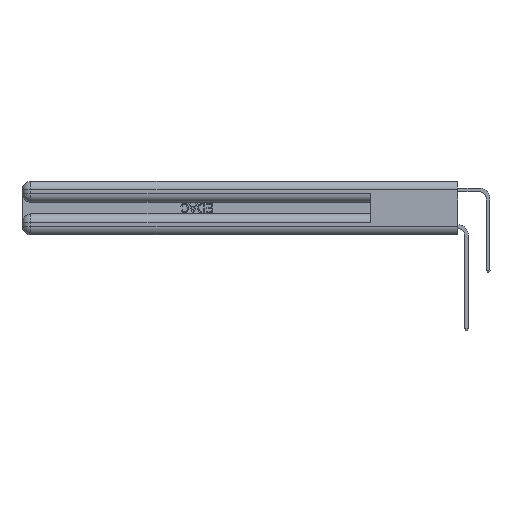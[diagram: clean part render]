
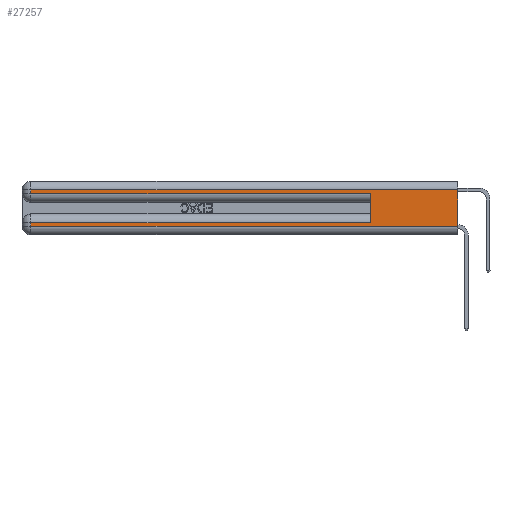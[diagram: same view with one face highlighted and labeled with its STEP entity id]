
A CAD part, left-side view. The second image highlights one B-rep face of the part: STEP entity #27257.
In plain terms, the highlighted planar face has unit normal (-1, 0, 0).
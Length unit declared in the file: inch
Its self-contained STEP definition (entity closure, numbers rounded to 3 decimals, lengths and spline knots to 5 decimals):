
#661 = VERTEX_POINT ( 'NONE', #8193 ) ;
#1344 = VERTEX_POINT ( 'NONE', #17011 ) ;
#1753 = CARTESIAN_POINT ( 'NONE',  ( 0., 2.94, 0.37 ) ) ;
#2162 = ORIENTED_EDGE ( 'NONE', *, *, #30334, .F. ) ;
#3228 = VECTOR ( 'NONE', #27298, 39.37008 ) ;
#3565 = VERTEX_POINT ( 'NONE', #12683 ) ;
#4190 = ORIENTED_EDGE ( 'NONE', *, *, #29912, .T. ) ;
#4237 = LINE ( 'NONE', #1753, #13322 ) ;
#4290 = CARTESIAN_POINT ( 'NONE',  ( 0., 0., 0.37 ) ) ;
#4573 = CARTESIAN_POINT ( 'NONE',  ( 0., 0.6, 0.285 ) ) ;
#5246 = CARTESIAN_POINT ( 'NONE',  ( 0., 2.94, 0.31 ) ) ;
#5286 = AXIS2_PLACEMENT_3D ( 'NONE', #32133, #14847, #19780 ) ;
#5303 = LINE ( 'NONE', #10839, #9142 ) ;
#5485 = CARTESIAN_POINT ( 'NONE',  ( 0., 0., 0.285 ) ) ;
#6929 = CARTESIAN_POINT ( 'NONE',  ( 0., 0., 0.31 ) ) ;
#7421 = CARTESIAN_POINT ( 'NONE',  ( 0., 0., 0.085 ) ) ;
#8007 = VERTEX_POINT ( 'NONE', #24613 ) ;
#8073 = ORIENTED_EDGE ( 'NONE', *, *, #30149, .T. ) ;
#8193 = CARTESIAN_POINT ( 'NONE',  ( 0., 0., 0.06 ) ) ;
#9142 = VECTOR ( 'NONE', #25018, 39.37008 ) ;
#10044 = DIRECTION ( 'NONE',  ( 0., 1., 0. ) ) ;
#10587 = VERTEX_POINT ( 'NONE', #27217 ) ;
#10736 = FACE_OUTER_BOUND ( 'NONE', #17680, .T. ) ;
#10839 = CARTESIAN_POINT ( 'NONE',  ( 0., 0.6, 0.145 ) ) ;
#11216 = EDGE_CURVE ( 'NONE', #8007, #10587, #24438, .T. ) ;
#11605 = VECTOR ( 'NONE', #14109, 39.37008 ) ;
#11697 = CARTESIAN_POINT ( 'NONE',  ( 0., 0., 0.06 ) ) ;
#12253 = PLANE ( 'NONE',  #5286 ) ;
#12683 = CARTESIAN_POINT ( 'NONE',  ( 0., 0., 0.31 ) ) ;
#12942 = VECTOR ( 'NONE', #24600, 39.37008 ) ;
#13322 = VECTOR ( 'NONE', #16979, 39.37008 ) ;
#14109 = DIRECTION ( 'NONE',  ( 0., -1., 0. ) ) ;
#14599 = LINE ( 'NONE', #11697, #11605 ) ;
#14847 = DIRECTION ( 'NONE',  ( 1., 0., 0. ) ) ;
#16370 = EDGE_CURVE ( 'NONE', #28521, #16563, #4237, .T. ) ;
#16563 = VERTEX_POINT ( 'NONE', #27838 ) ;
#16886 = LINE ( 'NONE', #4290, #25620 ) ;
#16979 = DIRECTION ( 'NONE',  ( 0., 0., -1. ) ) ;
#17011 = CARTESIAN_POINT ( 'NONE',  ( 0., 0.6, 0.085 ) ) ;
#17680 = EDGE_LOOP ( 'NONE', ( #17931, #8073, #31713, #4190, #2162, #29320, #31183, #22426 ) ) ;
#17931 = ORIENTED_EDGE ( 'NONE', *, *, #22039, .F. ) ;
#18615 = VECTOR ( 'NONE', #10044, 39.37008 ) ;
#19661 = VECTOR ( 'NONE', #25708, 39.37008 ) ;
#19780 = DIRECTION ( 'NONE',  ( 0., 0., -1. ) ) ;
#19978 = EDGE_CURVE ( 'NONE', #10587, #661, #14599, .T. ) ;
#22039 = EDGE_CURVE ( 'NONE', #3565, #661, #16886, .T. ) ;
#22426 = ORIENTED_EDGE ( 'NONE', *, *, #19978, .T. ) ;
#24342 = DIRECTION ( 'NONE',  ( 0., 0., -1. ) ) ;
#24438 = LINE ( 'NONE', #31805, #12942 ) ;
#24600 = DIRECTION ( 'NONE',  ( 0., 0., -1. ) ) ;
#24613 = CARTESIAN_POINT ( 'NONE',  ( 0., 2.94, 0.085 ) ) ;
#25018 = DIRECTION ( 'NONE',  ( 0., 0., 1. ) ) ;
#25620 = VECTOR ( 'NONE', #24342, 39.37008 ) ;
#25708 = DIRECTION ( 'NONE',  ( 0., -1., 0. ) ) ;
#26809 = LINE ( 'NONE', #6929, #18615 ) ;
#27217 = CARTESIAN_POINT ( 'NONE',  ( 0., 2.94, 0.06 ) ) ;
#27257 = ADVANCED_FACE ( 'NONE', ( #10736 ), #12253, .F. ) ;
#27298 = DIRECTION ( 'NONE',  ( 0., 1., 0. ) ) ;
#27838 = CARTESIAN_POINT ( 'NONE',  ( 0., 2.94, 0.285 ) ) ;
#27983 = LINE ( 'NONE', #5485, #19661 ) ;
#28521 = VERTEX_POINT ( 'NONE', #5246 ) ;
#29015 = EDGE_CURVE ( 'NONE', #1344, #8007, #29770, .T. ) ;
#29320 = ORIENTED_EDGE ( 'NONE', *, *, #29015, .T. ) ;
#29770 = LINE ( 'NONE', #7421, #3228 ) ;
#29912 = EDGE_CURVE ( 'NONE', #16563, #31123, #27983, .T. ) ;
#30149 = EDGE_CURVE ( 'NONE', #3565, #28521, #26809, .T. ) ;
#30334 = EDGE_CURVE ( 'NONE', #1344, #31123, #5303, .T. ) ;
#31123 = VERTEX_POINT ( 'NONE', #4573 ) ;
#31183 = ORIENTED_EDGE ( 'NONE', *, *, #11216, .T. ) ;
#31713 = ORIENTED_EDGE ( 'NONE', *, *, #16370, .T. ) ;
#31805 = CARTESIAN_POINT ( 'NONE',  ( 0., 2.94, 0.37 ) ) ;
#32133 = CARTESIAN_POINT ( 'NONE',  ( 0., 0., 0.37 ) ) ;
